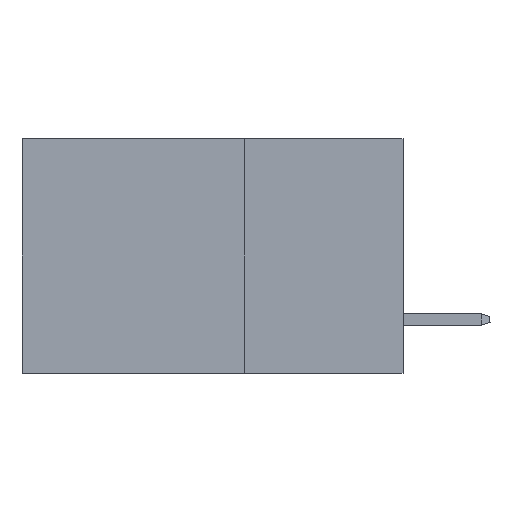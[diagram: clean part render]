
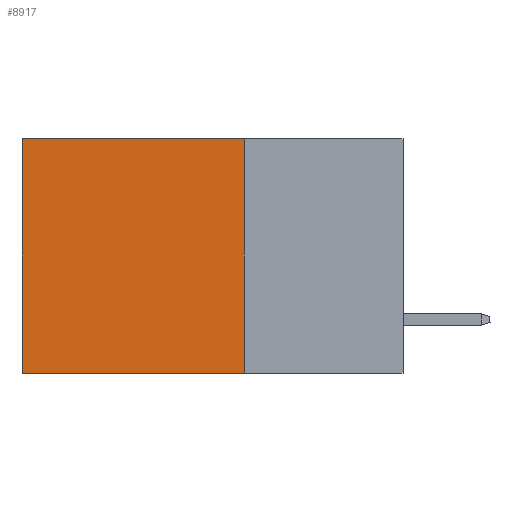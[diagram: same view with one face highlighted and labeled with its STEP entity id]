
A CAD part, left-side view. The second image highlights one B-rep face of the part: STEP entity #8917.
In plain terms, the highlighted planar face has unit normal (-1, 0, 0).
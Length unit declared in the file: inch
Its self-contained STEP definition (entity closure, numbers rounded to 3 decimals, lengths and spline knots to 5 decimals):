
#1875 = LINE ( 'NONE', #10529, #15468 ) ;
#2294 = PLANE ( 'NONE',  #26343 ) ;
#2432 = DIRECTION ( 'NONE',  ( 0., 0., -1. ) ) ;
#2898 = DIRECTION ( 'NONE',  ( 0., 1., 0. ) ) ;
#3348 = CARTESIAN_POINT ( 'NONE',  ( 0.2875, 0.6, -0.37 ) ) ;
#3393 = ORIENTED_EDGE ( 'NONE', *, *, #17983, .T. ) ;
#3973 = LINE ( 'NONE', #20968, #19915 ) ;
#4422 = DIRECTION ( 'NONE',  ( 1., 0., 0. ) ) ;
#4702 = VERTEX_POINT ( 'NONE', #3348 ) ;
#5887 = ORIENTED_EDGE ( 'NONE', *, *, #21999, .T. ) ;
#7581 = EDGE_CURVE ( 'NONE', #14365, #4702, #1875, .T. ) ;
#8108 = CARTESIAN_POINT ( 'NONE',  ( 0.2875, 0.25, 0. ) ) ;
#8917 = ADVANCED_FACE ( 'NONE', ( #25938 ), #2294, .F. ) ;
#9319 = ORIENTED_EDGE ( 'NONE', *, *, #7581, .F. ) ;
#10287 = VERTEX_POINT ( 'NONE', #25973 ) ;
#10529 = CARTESIAN_POINT ( 'NONE',  ( 0.2875, 0.25, -0.37 ) ) ;
#11539 = LINE ( 'NONE', #8108, #14164 ) ;
#11920 = EDGE_LOOP ( 'NONE', ( #3393, #9319, #24853, #5887 ) ) ;
#12125 = VECTOR ( 'NONE', #22139, 39.37008 ) ;
#12971 = CARTESIAN_POINT ( 'NONE',  ( 0.2875, 0.25, -0.37 ) ) ;
#13226 = CARTESIAN_POINT ( 'NONE',  ( 0.2875, 0.25, 0. ) ) ;
#13366 = LINE ( 'NONE', #13226, #12125 ) ;
#13390 = CARTESIAN_POINT ( 'NONE',  ( 0.2875, 0.6, 0. ) ) ;
#14164 = VECTOR ( 'NONE', #2898, 39.37008 ) ;
#14365 = VERTEX_POINT ( 'NONE', #12971 ) ;
#15468 = VECTOR ( 'NONE', #20726, 39.37008 ) ;
#16126 = EDGE_CURVE ( 'NONE', #10287, #14365, #13366, .T. ) ;
#16999 = DIRECTION ( 'NONE',  ( 0., 0., -1. ) ) ;
#17443 = CARTESIAN_POINT ( 'NONE',  ( 0.2875, 0.25, 0. ) ) ;
#17983 = EDGE_CURVE ( 'NONE', #24681, #4702, #3973, .T. ) ;
#19915 = VECTOR ( 'NONE', #16999, 39.37008 ) ;
#20726 = DIRECTION ( 'NONE',  ( 0., 1., 0. ) ) ;
#20968 = CARTESIAN_POINT ( 'NONE',  ( 0.2875, 0.6, 0. ) ) ;
#21999 = EDGE_CURVE ( 'NONE', #10287, #24681, #11539, .T. ) ;
#22139 = DIRECTION ( 'NONE',  ( 0., 0., -1. ) ) ;
#24681 = VERTEX_POINT ( 'NONE', #13390 ) ;
#24853 = ORIENTED_EDGE ( 'NONE', *, *, #16126, .F. ) ;
#25938 = FACE_OUTER_BOUND ( 'NONE', #11920, .T. ) ;
#25973 = CARTESIAN_POINT ( 'NONE',  ( 0.2875, 0.25, 0. ) ) ;
#26343 = AXIS2_PLACEMENT_3D ( 'NONE', #17443, #4422, #2432 ) ;
